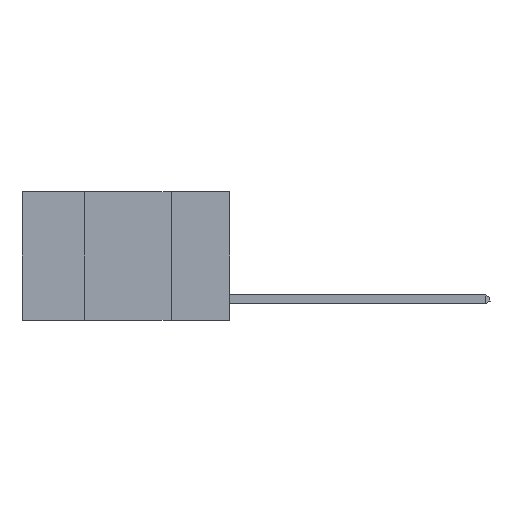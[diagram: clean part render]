
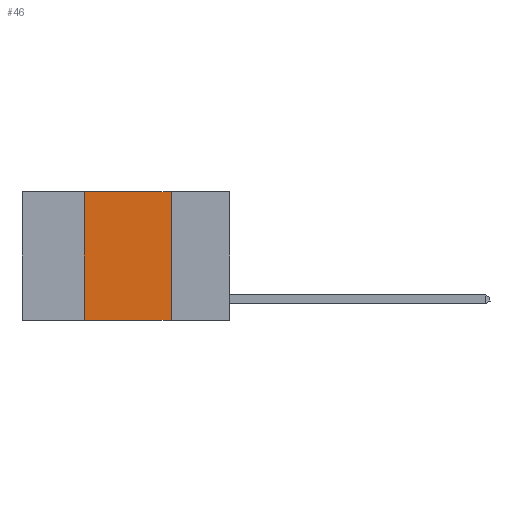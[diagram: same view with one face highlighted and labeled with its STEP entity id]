
A CAD part, left-side view. The second image highlights one B-rep face of the part: STEP entity #46.
In plain terms, the highlighted planar face has unit normal (-1, 0, 0).
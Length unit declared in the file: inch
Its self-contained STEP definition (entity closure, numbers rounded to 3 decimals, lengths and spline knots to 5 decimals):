
#46 = ADVANCED_FACE ( 'NONE', ( #9571 ), #15152, .F. ) ;
#62 = AXIS2_PLACEMENT_3D ( 'NONE', #5503, #6883, #16652 ) ;
#527 = DIRECTION ( 'NONE',  ( 0., 0., -1. ) ) ;
#619 = CARTESIAN_POINT ( 'NONE',  ( 0., 0.17, -0.37 ) ) ;
#779 = VECTOR ( 'NONE', #9151, 39.37008 ) ;
#1421 = EDGE_CURVE ( 'NONE', #8772, #3335, #7325, .T. ) ;
#1721 = DIRECTION ( 'NONE',  ( 0., -1., 0. ) ) ;
#2764 = CARTESIAN_POINT ( 'NONE',  ( 0., 0.6, 0. ) ) ;
#2948 = EDGE_LOOP ( 'NONE', ( #6729, #10183, #10112, #6405 ) ) ;
#3335 = VERTEX_POINT ( 'NONE', #12867 ) ;
#5503 = CARTESIAN_POINT ( 'NONE',  ( 0., 0.6, 0. ) ) ;
#6405 = ORIENTED_EDGE ( 'NONE', *, *, #8681, .T. ) ;
#6466 = VERTEX_POINT ( 'NONE', #619 ) ;
#6549 = LINE ( 'NONE', #16528, #16581 ) ;
#6729 = ORIENTED_EDGE ( 'NONE', *, *, #10823, .F. ) ;
#6883 = DIRECTION ( 'NONE',  ( 1., 0., 0. ) ) ;
#6939 = DIRECTION ( 'NONE',  ( 0., -1., 0. ) ) ;
#7325 = LINE ( 'NONE', #2764, #11027 ) ;
#8260 = VECTOR ( 'NONE', #1721, 39.37008 ) ;
#8681 = EDGE_CURVE ( 'NONE', #8684, #6466, #12404, .T. ) ;
#8684 = VERTEX_POINT ( 'NONE', #14247 ) ;
#8772 = VERTEX_POINT ( 'NONE', #14427 ) ;
#9151 = DIRECTION ( 'NONE',  ( 0., 0., 1. ) ) ;
#9571 = FACE_OUTER_BOUND ( 'NONE', #2948, .T. ) ;
#10112 = ORIENTED_EDGE ( 'NONE', *, *, #10223, .F. ) ;
#10183 = ORIENTED_EDGE ( 'NONE', *, *, #1421, .F. ) ;
#10223 = EDGE_CURVE ( 'NONE', #8684, #8772, #10902, .T. ) ;
#10823 = EDGE_CURVE ( 'NONE', #3335, #6466, #6549, .T. ) ;
#10902 = LINE ( 'NONE', #14502, #779 ) ;
#11027 = VECTOR ( 'NONE', #6939, 39.37008 ) ;
#12404 = LINE ( 'NONE', #15543, #8260 ) ;
#12867 = CARTESIAN_POINT ( 'NONE',  ( 0., 0.17, 0. ) ) ;
#14247 = CARTESIAN_POINT ( 'NONE',  ( 0., 0.42, -0.37 ) ) ;
#14427 = CARTESIAN_POINT ( 'NONE',  ( 0., 0.42, 0. ) ) ;
#14502 = CARTESIAN_POINT ( 'NONE',  ( 0., 0.42, 0. ) ) ;
#15152 = PLANE ( 'NONE',  #62 ) ;
#15543 = CARTESIAN_POINT ( 'NONE',  ( 0., 0.6, -0.37 ) ) ;
#16528 = CARTESIAN_POINT ( 'NONE',  ( 0., 0.17, 0. ) ) ;
#16581 = VECTOR ( 'NONE', #527, 39.37008 ) ;
#16652 = DIRECTION ( 'NONE',  ( 0., 0., -1. ) ) ;
